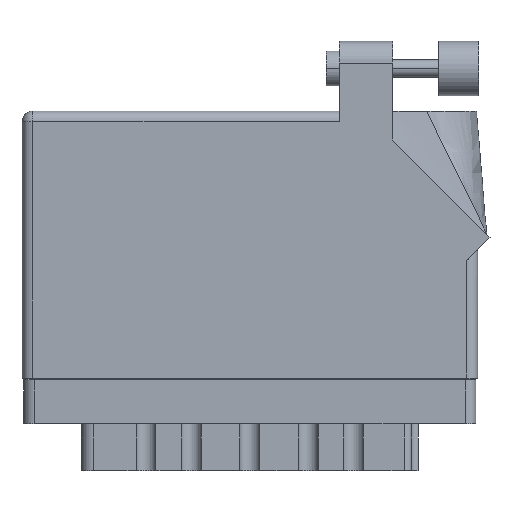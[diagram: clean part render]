
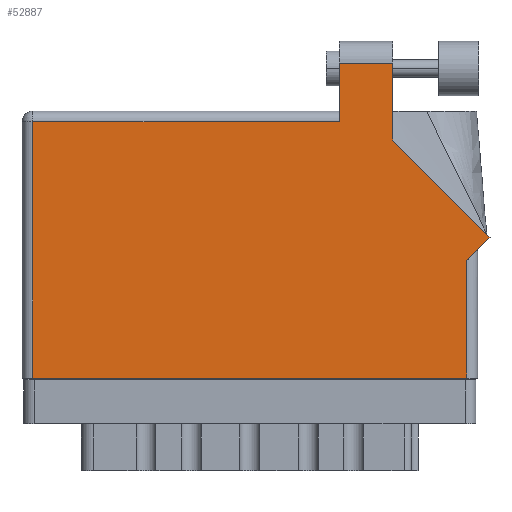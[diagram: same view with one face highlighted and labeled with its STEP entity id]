
A CAD part, front view. The second image highlights one B-rep face of the part: STEP entity #52887.
In plain terms, the highlighted face is planar.
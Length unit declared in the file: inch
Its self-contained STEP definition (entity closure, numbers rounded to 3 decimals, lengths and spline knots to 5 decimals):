
#1209 = CARTESIAN_POINT ( 'NONE',  ( 0., 0., 0. ) ) ;
#2402 = CARTESIAN_POINT ( 'NONE',  ( 1.819, 1.468, 0. ) ) ;
#2472 = VECTOR ( 'NONE', #41848, 39.37008 ) ;
#3069 = EDGE_CURVE ( 'NONE', #19203, #13402, #10554, .T. ) ;
#3429 = ORIENTED_EDGE ( 'NONE', *, *, #53048, .T. ) ;
#3636 = ORIENTED_EDGE ( 'NONE', *, *, #32288, .T. ) ;
#4111 = CARTESIAN_POINT ( 'NONE',  ( 2.68271, 0.80771, 0. ) ) ;
#7150 = CARTESIAN_POINT ( 'NONE',  ( 2.126, 1.36442, 0. ) ) ;
#7226 = VERTEX_POINT ( 'NONE', #7150 ) ;
#7504 = CARTESIAN_POINT ( 'NONE',  ( 1.819, 1.53, 0. ) ) ;
#7952 = CARTESIAN_POINT ( 'NONE',  ( 0.062, 0., 0. ) ) ;
#8032 = DIRECTION ( 'NONE',  ( 0., 1., 0. ) ) ;
#8324 = DIRECTION ( 'NONE',  ( 0., 1., 0. ) ) ;
#8396 = DIRECTION ( 'NONE',  ( 0.707, 0.707, 0. ) ) ;
#8652 = ORIENTED_EDGE ( 'NONE', *, *, #28340, .T. ) ;
#10554 = LINE ( 'NONE', #7952, #53262 ) ;
#11572 = PLANE ( 'NONE',  #42932 ) ;
#12015 = CARTESIAN_POINT ( 'NONE',  ( 1.819, 1.805, 0. ) ) ;
#12142 = VERTEX_POINT ( 'NONE', #2402 ) ;
#12239 = EDGE_LOOP ( 'NONE', ( #8652, #51866, #49462, #15491, #45391, #31268, #3429, #17759, #3636 ) ) ;
#13402 = VERTEX_POINT ( 'NONE', #36692 ) ;
#14249 = CARTESIAN_POINT ( 'NONE',  ( 2.68271, 0.80771, 0. ) ) ;
#15491 = ORIENTED_EDGE ( 'NONE', *, *, #36338, .T. ) ;
#15742 = VECTOR ( 'NONE', #8032, 39.37008 ) ;
#16032 = LINE ( 'NONE', #33797, #28277 ) ;
#17759 = ORIENTED_EDGE ( 'NONE', *, *, #35637, .T. ) ;
#19203 = VERTEX_POINT ( 'NONE', #30801 ) ;
#19349 = LINE ( 'NONE', #39137, #32918 ) ;
#20394 = LINE ( 'NONE', #7504, #30096 ) ;
#21421 = DIRECTION ( 'NONE',  ( 1., 0., 0. ) ) ;
#21898 = DIRECTION ( 'NONE',  ( -1., 0., 0. ) ) ;
#22536 = LINE ( 'NONE', #4111, #2472 ) ;
#23440 = DIRECTION ( 'NONE',  ( 0., -1., 0. ) ) ;
#26189 = EDGE_CURVE ( 'NONE', #13402, #45733, #46528, .T. ) ;
#27189 = LINE ( 'NONE', #29143, #44051 ) ;
#27583 = EDGE_CURVE ( 'NONE', #40822, #12142, #20394, .T. ) ;
#27826 = CARTESIAN_POINT ( 'NONE',  ( 0., 1.53, 0. ) ) ;
#28277 = VECTOR ( 'NONE', #21898, 39.37008 ) ;
#28340 = EDGE_CURVE ( 'NONE', #7226, #40875, #38441, .T. ) ;
#28524 = DIRECTION ( 'NONE',  ( 0., -1., 0. ) ) ;
#29143 = CARTESIAN_POINT ( 'NONE',  ( 2.612, 0.737, 0. ) ) ;
#29321 = FACE_OUTER_BOUND ( 'NONE', #12239, .T. ) ;
#30096 = VECTOR ( 'NONE', #23440, 39.37008 ) ;
#30801 = CARTESIAN_POINT ( 'NONE',  ( 0.062, 1.468, 0. ) ) ;
#30962 = VECTOR ( 'NONE', #21421, 39.37008 ) ;
#31268 = ORIENTED_EDGE ( 'NONE', *, *, #26189, .T. ) ;
#32288 = EDGE_CURVE ( 'NONE', #44973, #7226, #22536, .T. ) ;
#32494 = VECTOR ( 'NONE', #8324, 39.37008 ) ;
#32918 = VECTOR ( 'NONE', #38786, 39.37008 ) ;
#33797 = CARTESIAN_POINT ( 'NONE',  ( 0., 1.468, 0. ) ) ;
#35637 = EDGE_CURVE ( 'NONE', #52916, #44973, #27189, .T. ) ;
#36338 = EDGE_CURVE ( 'NONE', #12142, #19203, #16032, .T. ) ;
#36692 = CARTESIAN_POINT ( 'NONE',  ( 0.062, 0., 0. ) ) ;
#37058 = CARTESIAN_POINT ( 'NONE',  ( 2.55, 0.737, 0. ) ) ;
#38441 = LINE ( 'NONE', #40773, #15742 ) ;
#38786 = DIRECTION ( 'NONE',  ( -1., 0., 0. ) ) ;
#39137 = CARTESIAN_POINT ( 'NONE',  ( 1.819, 1.805, 0. ) ) ;
#40773 = CARTESIAN_POINT ( 'NONE',  ( 2.126, 1.36442, 0. ) ) ;
#40822 = VERTEX_POINT ( 'NONE', #12015 ) ;
#40875 = VERTEX_POINT ( 'NONE', #49837 ) ;
#41848 = DIRECTION ( 'NONE',  ( -0.707, 0.707, 0. ) ) ;
#42932 = AXIS2_PLACEMENT_3D ( 'NONE', #27826, #44503, #44692 ) ;
#43549 = LINE ( 'NONE', #37058, #32494 ) ;
#44051 = VECTOR ( 'NONE', #8396, 39.37008 ) ;
#44503 = DIRECTION ( 'NONE',  ( 0., 0., -1. ) ) ;
#44692 = DIRECTION ( 'NONE',  ( -1., 0., 0. ) ) ;
#44973 = VERTEX_POINT ( 'NONE', #14249 ) ;
#45321 = EDGE_CURVE ( 'NONE', #40875, #40822, #19349, .T. ) ;
#45391 = ORIENTED_EDGE ( 'NONE', *, *, #3069, .T. ) ;
#45733 = VERTEX_POINT ( 'NONE', #49414 ) ;
#45938 = CARTESIAN_POINT ( 'NONE',  ( 2.55, 0.675, 0. ) ) ;
#46528 = LINE ( 'NONE', #1209, #30962 ) ;
#49414 = CARTESIAN_POINT ( 'NONE',  ( 2.55, 0., 0. ) ) ;
#49462 = ORIENTED_EDGE ( 'NONE', *, *, #27583, .T. ) ;
#49837 = CARTESIAN_POINT ( 'NONE',  ( 2.126, 1.805, 0. ) ) ;
#51866 = ORIENTED_EDGE ( 'NONE', *, *, #45321, .T. ) ;
#52887 = ADVANCED_FACE ( 'NONE', ( #29321 ), #11572, .F. ) ;
#52916 = VERTEX_POINT ( 'NONE', #45938 ) ;
#53048 = EDGE_CURVE ( 'NONE', #45733, #52916, #43549, .T. ) ;
#53262 = VECTOR ( 'NONE', #28524, 39.37008 ) ;
